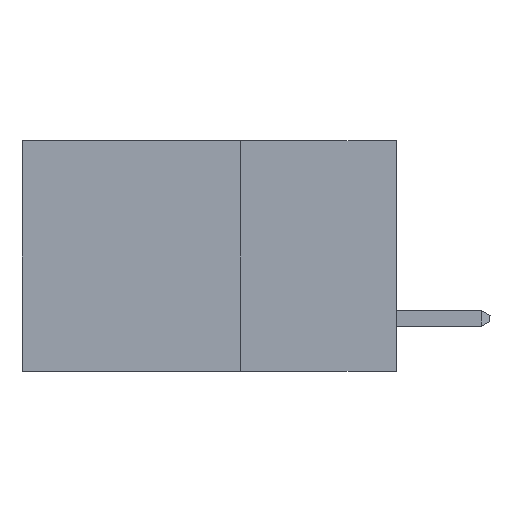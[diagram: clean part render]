
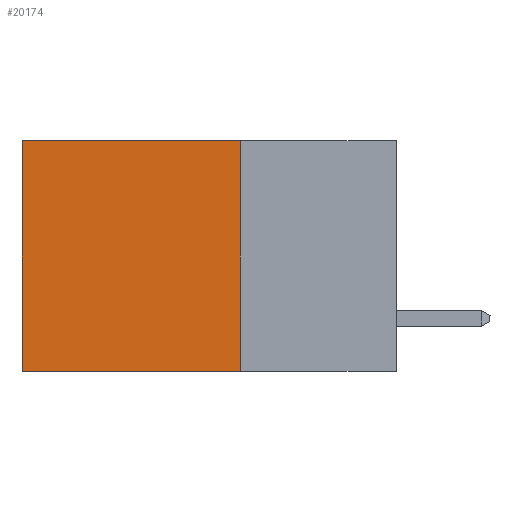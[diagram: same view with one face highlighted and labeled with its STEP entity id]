
A CAD part, left-side view. The second image highlights one B-rep face of the part: STEP entity #20174.
In plain terms, the highlighted planar face has unit normal (-1, 0, 0).
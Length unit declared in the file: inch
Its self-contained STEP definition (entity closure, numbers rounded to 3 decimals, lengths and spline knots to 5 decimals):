
#876 = EDGE_CURVE ( 'NONE', #13214, #9183, #18340, .T. ) ;
#896 = DIRECTION ( 'NONE',  ( 0., 1., 0. ) ) ;
#1122 = CARTESIAN_POINT ( 'NONE',  ( 0.2615, 0.25, -0.37 ) ) ;
#1486 = ORIENTED_EDGE ( 'NONE', *, *, #3978, .T. ) ;
#1642 = FACE_OUTER_BOUND ( 'NONE', #11071, .T. ) ;
#2786 = DIRECTION ( 'NONE',  ( 0., 0., -1. ) ) ;
#2830 = VECTOR ( 'NONE', #6409, 39.37008 ) ;
#3263 = ORIENTED_EDGE ( 'NONE', *, *, #3452, .F. ) ;
#3452 = EDGE_CURVE ( 'NONE', #11875, #13214, #19766, .T. ) ;
#3477 = AXIS2_PLACEMENT_3D ( 'NONE', #1122, #12421, #2786 ) ;
#3978 = EDGE_CURVE ( 'NONE', #11875, #16217, #6138, .T. ) ;
#4945 = EDGE_CURVE ( 'NONE', #16217, #9183, #19476, .T. ) ;
#5847 = CARTESIAN_POINT ( 'NONE',  ( 0.2615, 0.25, 0. ) ) ;
#5912 = DIRECTION ( 'NONE',  ( 0., 0., -1. ) ) ;
#6138 = LINE ( 'NONE', #5847, #2830 ) ;
#6409 = DIRECTION ( 'NONE',  ( 0., 1., 0. ) ) ;
#7146 = VECTOR ( 'NONE', #14375, 39.37008 ) ;
#7320 = VECTOR ( 'NONE', #5912, 39.37008 ) ;
#7583 = PLANE ( 'NONE',  #3477 ) ;
#9183 = VERTEX_POINT ( 'NONE', #9628 ) ;
#9628 = CARTESIAN_POINT ( 'NONE',  ( 0.2615, 0.6, -0.37 ) ) ;
#10126 = ORIENTED_EDGE ( 'NONE', *, *, #4945, .T. ) ;
#11071 = EDGE_LOOP ( 'NONE', ( #10126, #14628, #3263, #1486 ) ) ;
#11875 = VERTEX_POINT ( 'NONE', #12201 ) ;
#12201 = CARTESIAN_POINT ( 'NONE',  ( 0.2615, 0.25, 0. ) ) ;
#12421 = DIRECTION ( 'NONE',  ( 1., 0., 0. ) ) ;
#13214 = VERTEX_POINT ( 'NONE', #18540 ) ;
#13619 = VECTOR ( 'NONE', #896, 39.37008 ) ;
#14375 = DIRECTION ( 'NONE',  ( 0., 0., -1. ) ) ;
#14628 = ORIENTED_EDGE ( 'NONE', *, *, #876, .F. ) ;
#14772 = CARTESIAN_POINT ( 'NONE',  ( 0.2615, 0.25, -0.37 ) ) ;
#15507 = CARTESIAN_POINT ( 'NONE',  ( 0.2615, 0.6, -0.37 ) ) ;
#15771 = CARTESIAN_POINT ( 'NONE',  ( 0.2615, 0.25, -0.37 ) ) ;
#16217 = VERTEX_POINT ( 'NONE', #18833 ) ;
#18340 = LINE ( 'NONE', #15771, #13619 ) ;
#18540 = CARTESIAN_POINT ( 'NONE',  ( 0.2615, 0.25, -0.37 ) ) ;
#18833 = CARTESIAN_POINT ( 'NONE',  ( 0.2615, 0.6, 0. ) ) ;
#19476 = LINE ( 'NONE', #15507, #7320 ) ;
#19766 = LINE ( 'NONE', #14772, #7146 ) ;
#20174 = ADVANCED_FACE ( 'NONE', ( #1642 ), #7583, .F. ) ;
